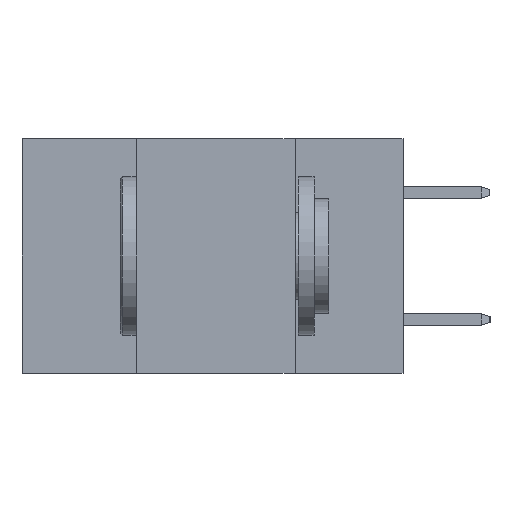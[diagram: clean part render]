
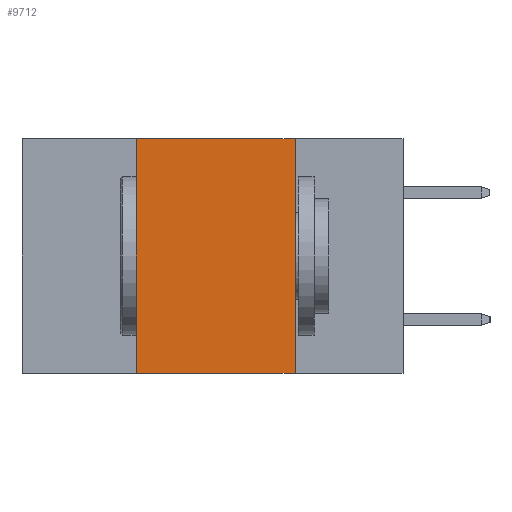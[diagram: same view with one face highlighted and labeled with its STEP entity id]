
A CAD part, left-side view. The second image highlights one B-rep face of the part: STEP entity #9712.
In plain terms, the highlighted planar face has unit normal (-1, 0, 0).
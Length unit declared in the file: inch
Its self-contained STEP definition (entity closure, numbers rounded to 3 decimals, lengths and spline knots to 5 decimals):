
#50 = VERTEX_POINT ( 'NONE', #9356 ) ;
#100 = LINE ( 'NONE', #9008, #2834 ) ;
#277 = AXIS2_PLACEMENT_3D ( 'NONE', #2148, #8470, #6143 ) ;
#417 = LINE ( 'NONE', #573, #1486 ) ;
#457 = ORIENTED_EDGE ( 'NONE', *, *, #9067, .F. ) ;
#573 = CARTESIAN_POINT ( 'NONE',  ( 0., 0.42, 0. ) ) ;
#1001 = DIRECTION ( 'NONE',  ( 0., 0., -1. ) ) ;
#1357 = DIRECTION ( 'NONE',  ( 0., -1., 0. ) ) ;
#1486 = VECTOR ( 'NONE', #3005, 39.37008 ) ;
#2052 = PLANE ( 'NONE',  #277 ) ;
#2148 = CARTESIAN_POINT ( 'NONE',  ( 0., 0.6, 0. ) ) ;
#2666 = VECTOR ( 'NONE', #1357, 39.37008 ) ;
#2834 = VECTOR ( 'NONE', #1001, 39.37008 ) ;
#2907 = LINE ( 'NONE', #5253, #2666 ) ;
#2920 = ORIENTED_EDGE ( 'NONE', *, *, #9306, .F. ) ;
#2925 = EDGE_CURVE ( 'NONE', #5040, #3990, #6745, .T. ) ;
#3005 = DIRECTION ( 'NONE',  ( 0., 0., 1. ) ) ;
#3990 = VERTEX_POINT ( 'NONE', #5964 ) ;
#4228 = DIRECTION ( 'NONE',  ( 0., -1., 0. ) ) ;
#5040 = VERTEX_POINT ( 'NONE', #7554 ) ;
#5253 = CARTESIAN_POINT ( 'NONE',  ( 0., 0.6, 0. ) ) ;
#5288 = FACE_OUTER_BOUND ( 'NONE', #9446, .T. ) ;
#5964 = CARTESIAN_POINT ( 'NONE',  ( 0., 0.17, -0.37 ) ) ;
#6104 = VECTOR ( 'NONE', #4228, 39.37008 ) ;
#6143 = DIRECTION ( 'NONE',  ( 0., 0., -1. ) ) ;
#6745 = LINE ( 'NONE', #7527, #6104 ) ;
#7125 = ORIENTED_EDGE ( 'NONE', *, *, #2925, .T. ) ;
#7222 = ORIENTED_EDGE ( 'NONE', *, *, #9319, .F. ) ;
#7527 = CARTESIAN_POINT ( 'NONE',  ( 0., 0.6, -0.37 ) ) ;
#7554 = CARTESIAN_POINT ( 'NONE',  ( 0., 0.42, -0.37 ) ) ;
#8470 = DIRECTION ( 'NONE',  ( 1., 0., 0. ) ) ;
#8792 = CARTESIAN_POINT ( 'NONE',  ( 0., 0.42, 0. ) ) ;
#9008 = CARTESIAN_POINT ( 'NONE',  ( 0., 0.17, 0. ) ) ;
#9067 = EDGE_CURVE ( 'NONE', #50, #3990, #100, .T. ) ;
#9306 = EDGE_CURVE ( 'NONE', #10226, #50, #2907, .T. ) ;
#9319 = EDGE_CURVE ( 'NONE', #5040, #10226, #417, .T. ) ;
#9356 = CARTESIAN_POINT ( 'NONE',  ( 0., 0.17, 0. ) ) ;
#9446 = EDGE_LOOP ( 'NONE', ( #457, #2920, #7222, #7125 ) ) ;
#9712 = ADVANCED_FACE ( 'NONE', ( #5288 ), #2052, .F. ) ;
#10226 = VERTEX_POINT ( 'NONE', #8792 ) ;
